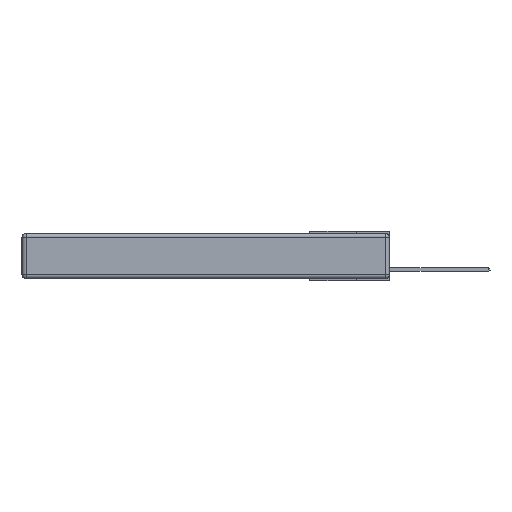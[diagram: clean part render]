
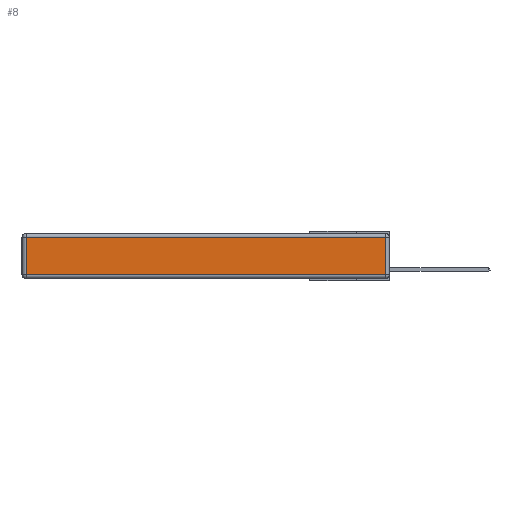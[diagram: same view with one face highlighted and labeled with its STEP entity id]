
A CAD part, left-side view. The second image highlights one B-rep face of the part: STEP entity #8.
In plain terms, the highlighted planar face has unit normal (-1, 0, 0).
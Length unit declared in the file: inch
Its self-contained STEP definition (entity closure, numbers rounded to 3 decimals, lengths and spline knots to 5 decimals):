
#8 = ADVANCED_FACE ( 'NONE', ( #2539 ), #14888, .T. ) ;
#254 = VECTOR ( 'NONE', #8933, 39.37008 ) ;
#914 = CARTESIAN_POINT ( 'NONE',  ( 0., 0.03, -0.343 ) ) ;
#2447 = VERTEX_POINT ( 'NONE', #13442 ) ;
#2539 = FACE_OUTER_BOUND ( 'NONE', #22420, .T. ) ;
#3137 = VERTEX_POINT ( 'NONE', #20628 ) ;
#3232 = LINE ( 'NONE', #21100, #21578 ) ;
#4406 = DIRECTION ( 'NONE',  ( 0., 0., 1. ) ) ;
#5189 = CARTESIAN_POINT ( 'NONE',  ( 0., 2.75, -0.03 ) ) ;
#6310 = EDGE_CURVE ( 'NONE', #10841, #21436, #14285, .T. ) ;
#6526 = AXIS2_PLACEMENT_3D ( 'NONE', #16749, #11459, #4406 ) ;
#6838 = CARTESIAN_POINT ( 'NONE',  ( 0., 0.03, -0.03 ) ) ;
#7698 = ORIENTED_EDGE ( 'NONE', *, *, #21546, .T. ) ;
#7902 = ORIENTED_EDGE ( 'NONE', *, *, #6310, .T. ) ;
#8933 = DIRECTION ( 'NONE',  ( 0., 0., -1. ) ) ;
#8952 = EDGE_CURVE ( 'NONE', #21436, #3137, #17480, .T. ) ;
#9094 = CARTESIAN_POINT ( 'NONE',  ( 0., 2.72, -0.343 ) ) ;
#9409 = ORIENTED_EDGE ( 'NONE', *, *, #11138, .T. ) ;
#10841 = VERTEX_POINT ( 'NONE', #13068 ) ;
#11138 = EDGE_CURVE ( 'NONE', #2447, #10841, #3232, .T. ) ;
#11459 = DIRECTION ( 'NONE',  ( -1., 0., 0. ) ) ;
#13068 = CARTESIAN_POINT ( 'NONE',  ( 0., 0.03, -0.313 ) ) ;
#13436 = ORIENTED_EDGE ( 'NONE', *, *, #8952, .T. ) ;
#13442 = CARTESIAN_POINT ( 'NONE',  ( 0., 2.72, -0.313 ) ) ;
#14285 = LINE ( 'NONE', #914, #18478 ) ;
#14888 = PLANE ( 'NONE',  #6526 ) ;
#16054 = DIRECTION ( 'NONE',  ( 0., 1., 0. ) ) ;
#16392 = VECTOR ( 'NONE', #16054, 39.37008 ) ;
#16749 = CARTESIAN_POINT ( 'NONE',  ( 0., 0., -0.343 ) ) ;
#17480 = LINE ( 'NONE', #5189, #16392 ) ;
#18478 = VECTOR ( 'NONE', #18577, 39.37008 ) ;
#18577 = DIRECTION ( 'NONE',  ( 0., 0., 1. ) ) ;
#19094 = LINE ( 'NONE', #9094, #254 ) ;
#20628 = CARTESIAN_POINT ( 'NONE',  ( 0., 2.72, -0.03 ) ) ;
#20947 = DIRECTION ( 'NONE',  ( 0., -1., 0. ) ) ;
#21100 = CARTESIAN_POINT ( 'NONE',  ( 0., 0., -0.313 ) ) ;
#21436 = VERTEX_POINT ( 'NONE', #6838 ) ;
#21546 = EDGE_CURVE ( 'NONE', #3137, #2447, #19094, .T. ) ;
#21578 = VECTOR ( 'NONE', #20947, 39.37008 ) ;
#22420 = EDGE_LOOP ( 'NONE', ( #9409, #7902, #13436, #7698 ) ) ;
